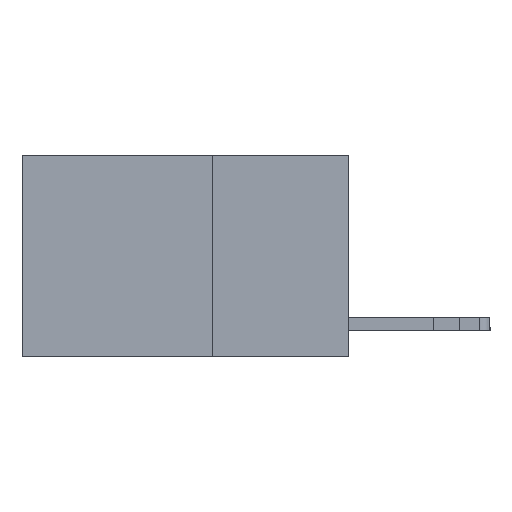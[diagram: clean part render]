
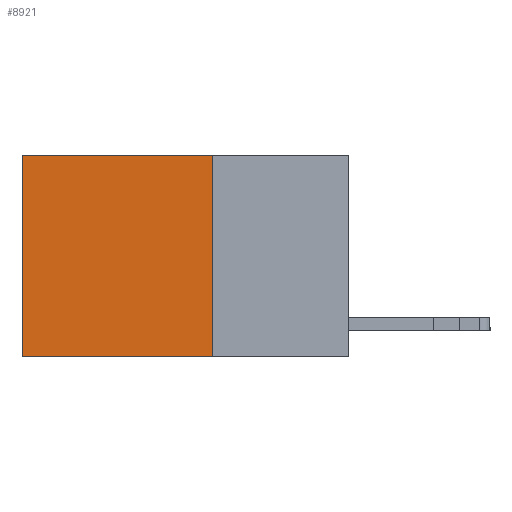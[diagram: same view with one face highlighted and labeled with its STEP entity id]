
A CAD part, left-side view. The second image highlights one B-rep face of the part: STEP entity #8921.
In plain terms, the highlighted planar face has unit normal (-1, 0, 0).
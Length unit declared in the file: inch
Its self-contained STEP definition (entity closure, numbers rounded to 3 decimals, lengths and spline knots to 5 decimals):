
#317 = DIRECTION ( 'NONE',  ( 0., 0., -1. ) ) ;
#430 = DIRECTION ( 'NONE',  ( 0., 0., -1. ) ) ;
#2065 = ORIENTED_EDGE ( 'NONE', *, *, #15894, .F. ) ;
#2720 = VERTEX_POINT ( 'NONE', #15061 ) ;
#2930 = VERTEX_POINT ( 'NONE', #16352 ) ;
#3046 = CARTESIAN_POINT ( 'NONE',  ( 0.2625, 0.6, 0. ) ) ;
#3207 = DIRECTION ( 'NONE',  ( 1., 0., 0. ) ) ;
#3811 = DIRECTION ( 'NONE',  ( 0., 1., 0. ) ) ;
#4298 = CARTESIAN_POINT ( 'NONE',  ( 0.2625, 0.6, 0. ) ) ;
#5024 = VECTOR ( 'NONE', #14936, 39.37008 ) ;
#5584 = LINE ( 'NONE', #11337, #13915 ) ;
#5854 = CARTESIAN_POINT ( 'NONE',  ( 0.2625, 0.25, 0. ) ) ;
#6059 = LINE ( 'NONE', #3046, #5024 ) ;
#6729 = CARTESIAN_POINT ( 'NONE',  ( 0.2625, 0.25, -0.37 ) ) ;
#8056 = VERTEX_POINT ( 'NONE', #4298 ) ;
#8528 = EDGE_CURVE ( 'NONE', #8056, #2930, #6059, .T. ) ;
#8921 = ADVANCED_FACE ( 'NONE', ( #14719 ), #16329, .F. ) ;
#9741 = LINE ( 'NONE', #6729, #12426 ) ;
#9758 = ORIENTED_EDGE ( 'NONE', *, *, #13864, .T. ) ;
#10473 = VERTEX_POINT ( 'NONE', #14331 ) ;
#10579 = EDGE_CURVE ( 'NONE', #2720, #10473, #17373, .T. ) ;
#11337 = CARTESIAN_POINT ( 'NONE',  ( 0.2625, 0.25, 0. ) ) ;
#12426 = VECTOR ( 'NONE', #3811, 39.37008 ) ;
#12782 = ORIENTED_EDGE ( 'NONE', *, *, #10579, .F. ) ;
#12943 = EDGE_LOOP ( 'NONE', ( #16194, #2065, #12782, #9758 ) ) ;
#13766 = AXIS2_PLACEMENT_3D ( 'NONE', #5854, #3207, #430 ) ;
#13864 = EDGE_CURVE ( 'NONE', #2720, #8056, #5584, .T. ) ;
#13915 = VECTOR ( 'NONE', #15687, 39.37008 ) ;
#14331 = CARTESIAN_POINT ( 'NONE',  ( 0.2625, 0.25, -0.37 ) ) ;
#14719 = FACE_OUTER_BOUND ( 'NONE', #12943, .T. ) ;
#14894 = CARTESIAN_POINT ( 'NONE',  ( 0.2625, 0.25, 0. ) ) ;
#14936 = DIRECTION ( 'NONE',  ( 0., 0., -1. ) ) ;
#15061 = CARTESIAN_POINT ( 'NONE',  ( 0.2625, 0.25, 0. ) ) ;
#15687 = DIRECTION ( 'NONE',  ( 0., 1., 0. ) ) ;
#15894 = EDGE_CURVE ( 'NONE', #10473, #2930, #9741, .T. ) ;
#16194 = ORIENTED_EDGE ( 'NONE', *, *, #8528, .T. ) ;
#16329 = PLANE ( 'NONE',  #13766 ) ;
#16352 = CARTESIAN_POINT ( 'NONE',  ( 0.2625, 0.6, -0.37 ) ) ;
#17143 = VECTOR ( 'NONE', #317, 39.37008 ) ;
#17373 = LINE ( 'NONE', #14894, #17143 ) ;
